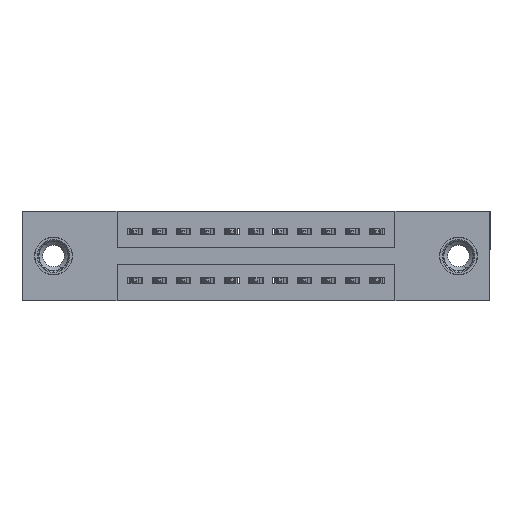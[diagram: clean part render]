
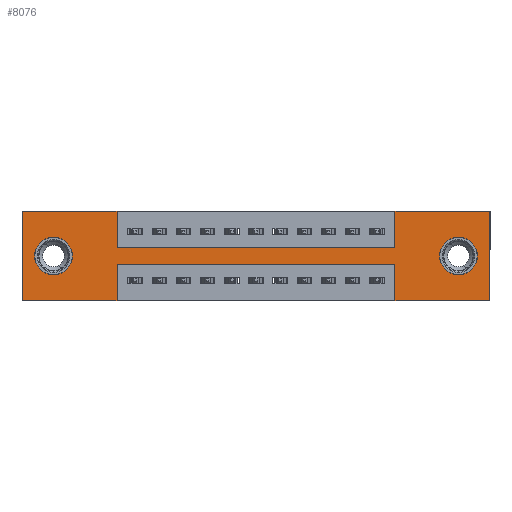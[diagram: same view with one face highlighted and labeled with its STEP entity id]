
A CAD part, front view. The second image highlights one B-rep face of the part: STEP entity #8076.
In plain terms, the highlighted planar face has unit normal (0, -1, 0).
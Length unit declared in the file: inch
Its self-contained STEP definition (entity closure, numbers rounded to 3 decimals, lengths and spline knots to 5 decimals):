
#36 = VERTEX_POINT ( 'NONE', #8661 ) ;
#107 = EDGE_CURVE ( 'NONE', #7021, #3414, #4659, .T. ) ;
#322 = VERTEX_POINT ( 'NONE', #8070 ) ;
#323 = VERTEX_POINT ( 'NONE', #2284 ) ;
#492 = DIRECTION ( 'NONE',  ( 0., 1., 0. ) ) ;
#704 = CARTESIAN_POINT ( 'NONE',  ( 1.5425, 0., -0.15 ) ) ;
#730 = DIRECTION ( 'NONE',  ( 1., 0., 0. ) ) ;
#807 = EDGE_CURVE ( 'NONE', #9572, #14851, #10800, .T. ) ;
#849 = CIRCLE ( 'NONE', #10112, 0.078 ) ;
#1136 = DIRECTION ( 'NONE',  ( -1., 0., 0. ) ) ;
#1489 = CARTESIAN_POINT ( 'NONE',  ( 1.935, 0., -0.37 ) ) ;
#1521 = EDGE_CURVE ( 'NONE', #2265, #8890, #5133, .T. ) ;
#1669 = VERTEX_POINT ( 'NONE', #1489 ) ;
#1922 = ORIENTED_EDGE ( 'NONE', *, *, #10229, .F. ) ;
#2265 = VERTEX_POINT ( 'NONE', #11644 ) ;
#2284 = CARTESIAN_POINT ( 'NONE',  ( 0., 0., -0.37 ) ) ;
#2427 = CARTESIAN_POINT ( 'NONE',  ( 0., 0., -0.37 ) ) ;
#2510 = ORIENTED_EDGE ( 'NONE', *, *, #6237, .F. ) ;
#2611 = CARTESIAN_POINT ( 'NONE',  ( 1.935, 0., 0. ) ) ;
#2951 = EDGE_CURVE ( 'NONE', #322, #3405, #14885, .T. ) ;
#2978 = CARTESIAN_POINT ( 'NONE',  ( 1.805, 0., -0.263 ) ) ;
#3083 = CARTESIAN_POINT ( 'NONE',  ( 1.5425, 0., 0. ) ) ;
#3217 = DIRECTION ( 'NONE',  ( 0., 0., -1. ) ) ;
#3310 = VECTOR ( 'NONE', #10805, 39.37008 ) ;
#3405 = VERTEX_POINT ( 'NONE', #3416 ) ;
#3414 = VERTEX_POINT ( 'NONE', #14899 ) ;
#3416 = CARTESIAN_POINT ( 'NONE',  ( 0.13, 0., -0.107 ) ) ;
#3422 = EDGE_CURVE ( 'NONE', #11861, #7021, #8490, .T. ) ;
#3523 = ORIENTED_EDGE ( 'NONE', *, *, #3422, .F. ) ;
#3642 = CARTESIAN_POINT ( 'NONE',  ( 1.805, 0., -0.107 ) ) ;
#3902 = CARTESIAN_POINT ( 'NONE',  ( 0.3925, 0., -0.37 ) ) ;
#4005 = CARTESIAN_POINT ( 'NONE',  ( 0., 0., -0.37 ) ) ;
#4119 = CARTESIAN_POINT ( 'NONE',  ( 0., 0., 0. ) ) ;
#4319 = LINE ( 'NONE', #4119, #11928 ) ;
#4346 = LINE ( 'NONE', #4707, #6318 ) ;
#4518 = CARTESIAN_POINT ( 'NONE',  ( 0.3925, 0., -0.15 ) ) ;
#4565 = CARTESIAN_POINT ( 'NONE',  ( 0., 0., -0.37 ) ) ;
#4625 = EDGE_LOOP ( 'NONE', ( #4866, #5663 ) ) ;
#4659 = LINE ( 'NONE', #3083, #9352 ) ;
#4707 = CARTESIAN_POINT ( 'NONE',  ( 1.5425, 0., -0.37 ) ) ;
#4713 = ORIENTED_EDGE ( 'NONE', *, *, #11386, .F. ) ;
#4812 = VECTOR ( 'NONE', #10768, 39.37008 ) ;
#4866 = ORIENTED_EDGE ( 'NONE', *, *, #14464, .T. ) ;
#4899 = VECTOR ( 'NONE', #13668, 39.37008 ) ;
#5133 = LINE ( 'NONE', #10770, #14388 ) ;
#5347 = ORIENTED_EDGE ( 'NONE', *, *, #7678, .T. ) ;
#5404 = ORIENTED_EDGE ( 'NONE', *, *, #5728, .F. ) ;
#5663 = ORIENTED_EDGE ( 'NONE', *, *, #2951, .T. ) ;
#5728 = EDGE_CURVE ( 'NONE', #7823, #11861, #12946, .T. ) ;
#5975 = LINE ( 'NONE', #12091, #9050 ) ;
#6009 = CARTESIAN_POINT ( 'NONE',  ( 0., 0., 0. ) ) ;
#6237 = EDGE_CURVE ( 'NONE', #8890, #323, #9124, .T. ) ;
#6318 = VECTOR ( 'NONE', #11696, 39.37008 ) ;
#6643 = CARTESIAN_POINT ( 'NONE',  ( 0., 0., 0. ) ) ;
#6810 = CARTESIAN_POINT ( 'NONE',  ( 1.5425, 0., -0.37 ) ) ;
#6830 = ORIENTED_EDGE ( 'NONE', *, *, #1521, .F. ) ;
#6884 = FACE_OUTER_BOUND ( 'NONE', #10168, .T. ) ;
#6897 = ORIENTED_EDGE ( 'NONE', *, *, #107, .F. ) ;
#7021 = VERTEX_POINT ( 'NONE', #704 ) ;
#7265 = EDGE_CURVE ( 'NONE', #36, #1669, #10185, .T. ) ;
#7292 = DIRECTION ( 'NONE',  ( 0., 0., -1. ) ) ;
#7405 = CARTESIAN_POINT ( 'NONE',  ( 0.13, 0., -0.185 ) ) ;
#7678 = EDGE_CURVE ( 'NONE', #14851, #9572, #8511, .T. ) ;
#7823 = VERTEX_POINT ( 'NONE', #8814 ) ;
#7849 = EDGE_LOOP ( 'NONE', ( #5347, #9143 ) ) ;
#7912 = VERTEX_POINT ( 'NONE', #6643 ) ;
#8070 = CARTESIAN_POINT ( 'NONE',  ( 0.13, 0., -0.263 ) ) ;
#8076 = ADVANCED_FACE ( 'NONE', ( #13394, #12685, #6884 ), #13944, .T. ) ;
#8316 = CARTESIAN_POINT ( 'NONE',  ( 0.3925, 0., -0.22 ) ) ;
#8441 = DIRECTION ( 'NONE',  ( -1., 0., 0. ) ) ;
#8490 = LINE ( 'NONE', #4518, #4899 ) ;
#8500 = LINE ( 'NONE', #6009, #11805 ) ;
#8511 = CIRCLE ( 'NONE', #9695, 0.078 ) ;
#8545 = DIRECTION ( 'NONE',  ( 0., 0., 1. ) ) ;
#8661 = CARTESIAN_POINT ( 'NONE',  ( 1.935, 0., 0. ) ) ;
#8682 = ORIENTED_EDGE ( 'NONE', *, *, #9288, .F. ) ;
#8696 = EDGE_CURVE ( 'NONE', #323, #7912, #8500, .T. ) ;
#8814 = CARTESIAN_POINT ( 'NONE',  ( 0.3925, 0., 0. ) ) ;
#8890 = VERTEX_POINT ( 'NONE', #3902 ) ;
#9050 = VECTOR ( 'NONE', #13186, 39.37008 ) ;
#9064 = VECTOR ( 'NONE', #1136, 39.37008 ) ;
#9124 = LINE ( 'NONE', #4005, #12575 ) ;
#9143 = ORIENTED_EDGE ( 'NONE', *, *, #807, .T. ) ;
#9288 = EDGE_CURVE ( 'NONE', #14722, #13340, #4346, .T. ) ;
#9352 = VECTOR ( 'NONE', #12423, 39.37008 ) ;
#9572 = VERTEX_POINT ( 'NONE', #2978 ) ;
#9632 = ORIENTED_EDGE ( 'NONE', *, *, #12203, .F. ) ;
#9695 = AXIS2_PLACEMENT_3D ( 'NONE', #12230, #10061, #12279 ) ;
#10023 = AXIS2_PLACEMENT_3D ( 'NONE', #2427, #10508, #11673 ) ;
#10061 = DIRECTION ( 'NONE',  ( 0., 1., 0. ) ) ;
#10112 = AXIS2_PLACEMENT_3D ( 'NONE', #10949, #13137, #13084 ) ;
#10168 = EDGE_LOOP ( 'NONE', ( #6830, #9632, #8682, #4713, #14206, #1922, #6897, #3523, #5404, #11319, #10359, #2510 ) ) ;
#10185 = LINE ( 'NONE', #2611, #3310 ) ;
#10229 = EDGE_CURVE ( 'NONE', #3414, #36, #4319, .T. ) ;
#10359 = ORIENTED_EDGE ( 'NONE', *, *, #8696, .F. ) ;
#10508 = DIRECTION ( 'NONE',  ( 0., -1., 0. ) ) ;
#10542 = DIRECTION ( 'NONE',  ( 0., 0., 1. ) ) ;
#10768 = DIRECTION ( 'NONE',  ( 0., 0., -1. ) ) ;
#10770 = CARTESIAN_POINT ( 'NONE',  ( 0.3925, 0., -0.37 ) ) ;
#10800 = CIRCLE ( 'NONE', #12567, 0.078 ) ;
#10805 = DIRECTION ( 'NONE',  ( 0., 0., -1. ) ) ;
#10853 = AXIS2_PLACEMENT_3D ( 'NONE', #7405, #492, #8545 ) ;
#10949 = CARTESIAN_POINT ( 'NONE',  ( 0.13, 0., -0.185 ) ) ;
#11254 = VECTOR ( 'NONE', #12882, 39.37008 ) ;
#11319 = ORIENTED_EDGE ( 'NONE', *, *, #11768, .F. ) ;
#11386 = EDGE_CURVE ( 'NONE', #1669, #14722, #13780, .T. ) ;
#11644 = CARTESIAN_POINT ( 'NONE',  ( 0.3925, 0., -0.22 ) ) ;
#11673 = DIRECTION ( 'NONE',  ( 0., 0., -1. ) ) ;
#11696 = DIRECTION ( 'NONE',  ( 0., 0., 1. ) ) ;
#11768 = EDGE_CURVE ( 'NONE', #7912, #7823, #5975, .T. ) ;
#11805 = VECTOR ( 'NONE', #10542, 39.37008 ) ;
#11861 = VERTEX_POINT ( 'NONE', #12137 ) ;
#11928 = VECTOR ( 'NONE', #730, 39.37008 ) ;
#12091 = CARTESIAN_POINT ( 'NONE',  ( 0., 0., 0. ) ) ;
#12137 = CARTESIAN_POINT ( 'NONE',  ( 0.3925, 0., -0.15 ) ) ;
#12203 = EDGE_CURVE ( 'NONE', #13340, #2265, #13022, .T. ) ;
#12230 = CARTESIAN_POINT ( 'NONE',  ( 1.805, 0., -0.185 ) ) ;
#12279 = DIRECTION ( 'NONE',  ( 0., 0., -1. ) ) ;
#12358 = DIRECTION ( 'NONE',  ( 0., 1., 0. ) ) ;
#12423 = DIRECTION ( 'NONE',  ( 0., 0., 1. ) ) ;
#12567 = AXIS2_PLACEMENT_3D ( 'NONE', #14800, #12358, #3217 ) ;
#12575 = VECTOR ( 'NONE', #8441, 39.37008 ) ;
#12685 = FACE_BOUND ( 'NONE', #4625, .T. ) ;
#12882 = DIRECTION ( 'NONE',  ( -1., 0., 0. ) ) ;
#12946 = LINE ( 'NONE', #13056, #4812 ) ;
#13022 = LINE ( 'NONE', #8316, #11254 ) ;
#13056 = CARTESIAN_POINT ( 'NONE',  ( 0.3925, 0., 0. ) ) ;
#13084 = DIRECTION ( 'NONE',  ( 0., 0., 1. ) ) ;
#13137 = DIRECTION ( 'NONE',  ( 0., 1., 0. ) ) ;
#13186 = DIRECTION ( 'NONE',  ( 1., 0., 0. ) ) ;
#13340 = VERTEX_POINT ( 'NONE', #14909 ) ;
#13394 = FACE_BOUND ( 'NONE', #7849, .T. ) ;
#13668 = DIRECTION ( 'NONE',  ( 1., 0., 0. ) ) ;
#13780 = LINE ( 'NONE', #4565, #9064 ) ;
#13944 = PLANE ( 'NONE',  #10023 ) ;
#14206 = ORIENTED_EDGE ( 'NONE', *, *, #7265, .F. ) ;
#14388 = VECTOR ( 'NONE', #7292, 39.37008 ) ;
#14464 = EDGE_CURVE ( 'NONE', #3405, #322, #849, .T. ) ;
#14722 = VERTEX_POINT ( 'NONE', #6810 ) ;
#14800 = CARTESIAN_POINT ( 'NONE',  ( 1.805, 0., -0.185 ) ) ;
#14851 = VERTEX_POINT ( 'NONE', #3642 ) ;
#14885 = CIRCLE ( 'NONE', #10853, 0.078 ) ;
#14899 = CARTESIAN_POINT ( 'NONE',  ( 1.5425, 0., 0. ) ) ;
#14909 = CARTESIAN_POINT ( 'NONE',  ( 1.5425, 0., -0.22 ) ) ;
